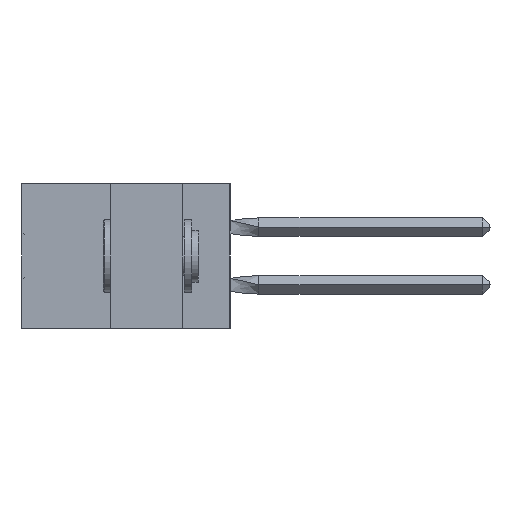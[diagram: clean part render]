
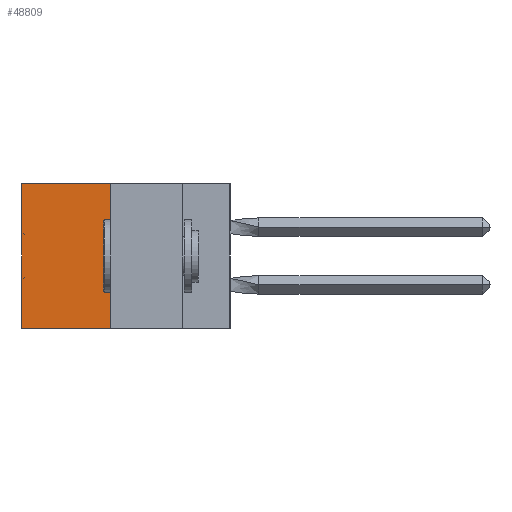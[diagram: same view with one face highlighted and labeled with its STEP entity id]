
A CAD part, left-side view. The second image highlights one B-rep face of the part: STEP entity #48809.
In plain terms, the highlighted planar face has unit normal (-1, 0, 0).
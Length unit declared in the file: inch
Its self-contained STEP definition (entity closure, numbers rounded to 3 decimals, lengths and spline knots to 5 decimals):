
#93 = CARTESIAN_POINT ( 'NONE',  ( 0.305, 0.72, -0.5 ) ) ;
#751 = EDGE_CURVE ( 'NONE', #42903, #7965, #28089, .T. ) ;
#4573 = EDGE_CURVE ( 'NONE', #29582, #42903, #22815, .T. ) ;
#5543 = AXIS2_PLACEMENT_3D ( 'NONE', #29890, #29710, #5935 ) ;
#5928 = CARTESIAN_POINT ( 'NONE',  ( 0.305, 0.72, -0.5 ) ) ;
#5935 = DIRECTION ( 'NONE',  ( 0., 0., -1. ) ) ;
#6919 = CARTESIAN_POINT ( 'NONE',  ( 0.305, 0.413, -0.5 ) ) ;
#7965 = VERTEX_POINT ( 'NONE', #93 ) ;
#13626 = PLANE ( 'NONE',  #5543 ) ;
#14138 = FACE_OUTER_BOUND ( 'NONE', #30894, .T. ) ;
#14212 = VERTEX_POINT ( 'NONE', #34334 ) ;
#15198 = DIRECTION ( 'NONE',  ( 0., 0., -1. ) ) ;
#15579 = ORIENTED_EDGE ( 'NONE', *, *, #43102, .T. ) ;
#18889 = EDGE_CURVE ( 'NONE', #14212, #7965, #47116, .T. ) ;
#20095 = CARTESIAN_POINT ( 'NONE',  ( 0.305, 0.413, 0. ) ) ;
#22815 = LINE ( 'NONE', #46704, #45578 ) ;
#23577 = ORIENTED_EDGE ( 'NONE', *, *, #751, .F. ) ;
#23822 = CARTESIAN_POINT ( 'NONE',  ( 0.305, 0.413, 0. ) ) ;
#24935 = VECTOR ( 'NONE', #24964, 39.37008 ) ;
#24964 = DIRECTION ( 'NONE',  ( 0., 0., -1. ) ) ;
#28089 = LINE ( 'NONE', #42324, #37335 ) ;
#29097 = VECTOR ( 'NONE', #39947, 39.37008 ) ;
#29582 = VERTEX_POINT ( 'NONE', #20095 ) ;
#29710 = DIRECTION ( 'NONE',  ( 1., 0., 0. ) ) ;
#29890 = CARTESIAN_POINT ( 'NONE',  ( 0.305, 0.413, -0.5 ) ) ;
#30385 = DIRECTION ( 'NONE',  ( 0., 1., 0. ) ) ;
#30894 = EDGE_LOOP ( 'NONE', ( #44329, #23577, #47265, #15579 ) ) ;
#34334 = CARTESIAN_POINT ( 'NONE',  ( 0.305, 0.72, 0. ) ) ;
#37335 = VECTOR ( 'NONE', #30385, 39.37008 ) ;
#39598 = LINE ( 'NONE', #23822, #29097 ) ;
#39947 = DIRECTION ( 'NONE',  ( 0., 1., 0. ) ) ;
#42324 = CARTESIAN_POINT ( 'NONE',  ( 0.305, 0.413, -0.5 ) ) ;
#42903 = VERTEX_POINT ( 'NONE', #6919 ) ;
#43102 = EDGE_CURVE ( 'NONE', #29582, #14212, #39598, .T. ) ;
#44329 = ORIENTED_EDGE ( 'NONE', *, *, #18889, .T. ) ;
#45578 = VECTOR ( 'NONE', #15198, 39.37008 ) ;
#46704 = CARTESIAN_POINT ( 'NONE',  ( 0.305, 0.413, -0.5 ) ) ;
#47116 = LINE ( 'NONE', #5928, #24935 ) ;
#47265 = ORIENTED_EDGE ( 'NONE', *, *, #4573, .F. ) ;
#48809 = ADVANCED_FACE ( 'NONE', ( #14138 ), #13626, .F. ) ;
